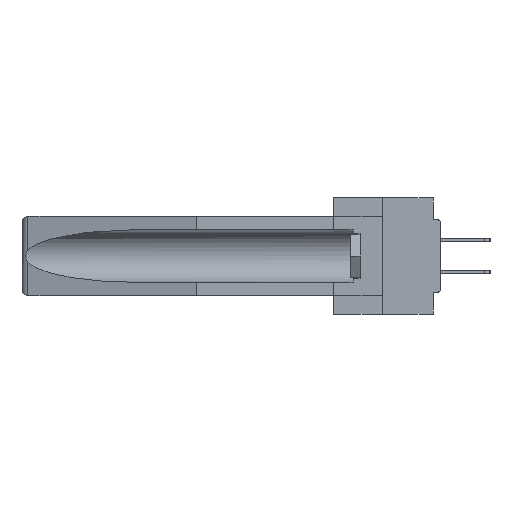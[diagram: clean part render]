
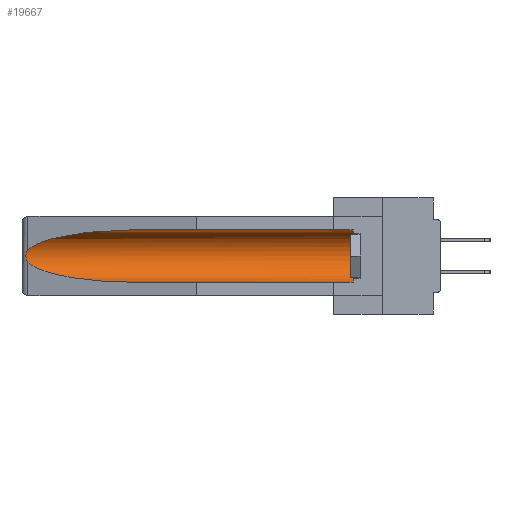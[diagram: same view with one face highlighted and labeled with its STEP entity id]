
A CAD part, left-side view. The second image highlights one B-rep face of the part: STEP entity #19667.
In plain terms, the highlighted cylindrical face has radius 2.857 mm (diameter 5.715 mm), a partial arc.
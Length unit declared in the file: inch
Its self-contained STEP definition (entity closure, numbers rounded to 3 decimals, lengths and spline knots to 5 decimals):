
#8 =( BOUNDED_CURVE ( )  B_SPLINE_CURVE ( 3, ( #968, #12430, #6550, #26010 ),
 .UNSPECIFIED., .F., .T. ) 
 B_SPLINE_CURVE_WITH_KNOTS ( ( 4, 4 ),
 ( 4.71239, 6.08839 ),
 .UNSPECIFIED. ) 
 CURVE ( )  GEOMETRIC_REPRESENTATION_ITEM ( )  RATIONAL_B_SPLINE_CURVE ( ( 1., 0.848, 0.848, 1. ) ) 
 REPRESENTATION_ITEM ( '' )  );
#968 = CARTESIAN_POINT ( 'NONE',  ( 0.155, 1.07973, -0.059 ) ) ;
#1702 = EDGE_CURVE ( 'NONE', #14374, #33995, #11496, .T. ) ;
#1874 = CARTESIAN_POINT ( 'NONE',  ( 0.26597, 1.5296, -0.19026 ) ) ;
#2690 = DIRECTION ( 'NONE',  ( 0., -1., 0. ) ) ;
#3172 = ORIENTED_EDGE ( 'NONE', *, *, #1702, .F. ) ;
#3269 = ORIENTED_EDGE ( 'NONE', *, *, #18624, .T. ) ;
#4343 = EDGE_CURVE ( 'NONE', #16952, #32516, #25282, .T. ) ;
#5980 = DIRECTION ( 'NONE',  ( 0., 1., 0. ) ) ;
#6483 = B_SPLINE_CURVE_WITH_KNOTS ( 'NONE', 3,
 ( #15908, #15785, #35395, #18604, #24450, #35659, #10493, #18844, #1874, #24203 ),
 .UNSPECIFIED., .F., .F.,
 ( 4, 2, 2, 2, 4 ),
 ( 0., 0.00029, 0.00058, 0.00087, 0.00117 ),
 .UNSPECIFIED. ) ;
#6550 = CARTESIAN_POINT ( 'NONE',  ( 0.25451, 1.48313, -0.09465 ) ) ;
#7070 = CIRCLE ( 'NONE', #26992, 0.1125 ) ;
#8228 = DIRECTION ( 'NONE',  ( 0., 1., 0. ) ) ;
#8876 = EDGE_CURVE ( 'NONE', #27015, #33995, #30920, .T. ) ;
#9106 = VECTOR ( 'NONE', #15370, 39.37008 ) ;
#10493 = CARTESIAN_POINT ( 'NONE',  ( 0.2673, 1.53269, -0.17917 ) ) ;
#11496 = LINE ( 'NONE', #31565, #18524 ) ;
#12430 = CARTESIAN_POINT ( 'NONE',  ( 0.21114, 1.30732, -0.059 ) ) ;
#13332 = CARTESIAN_POINT ( 'NONE',  ( 0.21114, 1.30732, -0.284 ) ) ;
#13391 = ORIENTED_EDGE ( 'NONE', *, *, #25717, .T. ) ;
#13836 = DIRECTION ( 'NONE',  ( 0., 0., 1. ) ) ;
#14366 = ORIENTED_EDGE ( 'NONE', *, *, #8876, .T. ) ;
#14374 = VERTEX_POINT ( 'NONE', #20911 ) ;
#15245 = CARTESIAN_POINT ( 'NONE',  ( 0.155, -0.30754, -0.059 ) ) ;
#15370 = DIRECTION ( 'NONE',  ( 0., 1., 0. ) ) ;
#15785 = CARTESIAN_POINT ( 'NONE',  ( 0.26597, 1.52961, -0.15275 ) ) ;
#15908 = CARTESIAN_POINT ( 'NONE',  ( 0.26537, 1.52718, -0.14972 ) ) ;
#16114 = CARTESIAN_POINT ( 'NONE',  ( 0.155, 1.07973, -0.284 ) ) ;
#16116 = ORIENTED_EDGE ( 'NONE', *, *, #16774, .T. ) ;
#16162 = EDGE_LOOP ( 'NONE', ( #3269, #16116, #14366, #3172, #13391, #33706 ) ) ;
#16740 = FACE_OUTER_BOUND ( 'NONE', #16162, .T. ) ;
#16774 = EDGE_CURVE ( 'NONE', #35027, #27015, #6483, .T. ) ;
#16952 = VERTEX_POINT ( 'NONE', #29605 ) ;
#18524 = VECTOR ( 'NONE', #5980, 39.37008 ) ;
#18604 = CARTESIAN_POINT ( 'NONE',  ( 0.2673, 1.5327, -0.16383 ) ) ;
#18624 = EDGE_CURVE ( 'NONE', #32516, #35027, #8, .T. ) ;
#18844 = CARTESIAN_POINT ( 'NONE',  ( 0.26655, 1.53094, -0.18657 ) ) ;
#18948 = CARTESIAN_POINT ( 'NONE',  ( 0.25451, 1.48313, -0.24835 ) ) ;
#19667 = ADVANCED_FACE ( 'NONE', ( #16740 ), #27676, .F. ) ;
#20911 = CARTESIAN_POINT ( 'NONE',  ( 0.155, 0.126, -0.284 ) ) ;
#21194 = CARTESIAN_POINT ( 'NONE',  ( 0.26537, 1.52718, -0.19328 ) ) ;
#22085 = DIRECTION ( 'NONE',  ( 0., 0., 1. ) ) ;
#22641 = CARTESIAN_POINT ( 'NONE',  ( 0.155, 1.07973, -0.284 ) ) ;
#24203 = CARTESIAN_POINT ( 'NONE',  ( 0.26537, 1.52718, -0.19328 ) ) ;
#24450 = CARTESIAN_POINT ( 'NONE',  ( 0.2675, 1.53308, -0.16763 ) ) ;
#25282 = LINE ( 'NONE', #15245, #9106 ) ;
#25717 = EDGE_CURVE ( 'NONE', #14374, #16952, #7070, .T. ) ;
#26010 = CARTESIAN_POINT ( 'NONE',  ( 0.26537, 1.52718, -0.14972 ) ) ;
#26992 = AXIS2_PLACEMENT_3D ( 'NONE', #30587, #2690, #13836 ) ;
#27015 = VERTEX_POINT ( 'NONE', #21194 ) ;
#27032 = CARTESIAN_POINT ( 'NONE',  ( 0.155, 1.07973, -0.059 ) ) ;
#27303 = AXIS2_PLACEMENT_3D ( 'NONE', #33246, #8228, #22085 ) ;
#27676 = CYLINDRICAL_SURFACE ( 'NONE', #27303, 0.1125 ) ;
#29605 = CARTESIAN_POINT ( 'NONE',  ( 0.155, 0.126, -0.059 ) ) ;
#30587 = CARTESIAN_POINT ( 'NONE',  ( 0.155, 0.126, -0.1715 ) ) ;
#30920 =( BOUNDED_CURVE ( )  B_SPLINE_CURVE ( 3, ( #32898, #18948, #13332, #16114 ),
 .UNSPECIFIED., .F., .F. ) 
 B_SPLINE_CURVE_WITH_KNOTS ( ( 4, 4 ),
 ( 0.1948, 1.5708 ),
 .UNSPECIFIED. ) 
 CURVE ( )  GEOMETRIC_REPRESENTATION_ITEM ( )  RATIONAL_B_SPLINE_CURVE ( ( 1., 0.848, 0.848, 1. ) ) 
 REPRESENTATION_ITEM ( '' )  );
#31565 = CARTESIAN_POINT ( 'NONE',  ( 0.155, -0.30754, -0.284 ) ) ;
#32516 = VERTEX_POINT ( 'NONE', #27032 ) ;
#32898 = CARTESIAN_POINT ( 'NONE',  ( 0.26537, 1.52718, -0.19328 ) ) ;
#33246 = CARTESIAN_POINT ( 'NONE',  ( 0.155, -0.30754, -0.1715 ) ) ;
#33706 = ORIENTED_EDGE ( 'NONE', *, *, #4343, .T. ) ;
#33904 = CARTESIAN_POINT ( 'NONE',  ( 0.26537, 1.52718, -0.14972 ) ) ;
#33995 = VERTEX_POINT ( 'NONE', #22641 ) ;
#35027 = VERTEX_POINT ( 'NONE', #33904 ) ;
#35395 = CARTESIAN_POINT ( 'NONE',  ( 0.26654, 1.53092, -0.15636 ) ) ;
#35659 = CARTESIAN_POINT ( 'NONE',  ( 0.2675, 1.53308, -0.17534 ) ) ;
